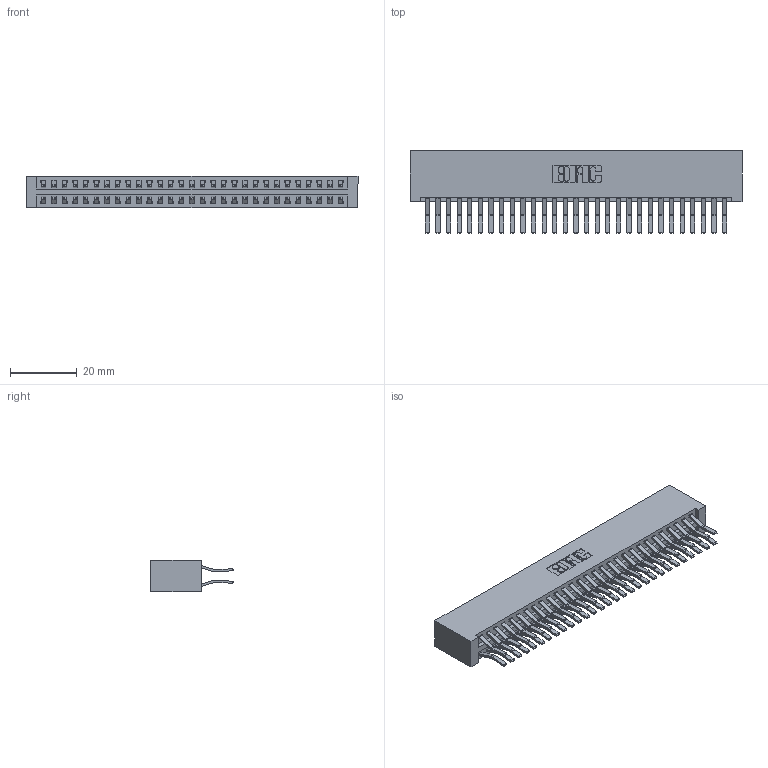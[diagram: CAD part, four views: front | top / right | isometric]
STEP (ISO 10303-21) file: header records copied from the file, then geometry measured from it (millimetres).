
FILE_DESCRIPTION (( 'STEP AP203' ), '1' );
FILE_NAME ('346-058-560-201.STEP', '2022-05-21T09:47:39', ( '' ), ( '' ), 'SwSTEP 2.0', 'SolidWorks 2020', '' );
FILE_SCHEMA (( 'CONFIG_CONTROL_DESIGN' ));
Length unit declared in the file: inch
Products named in the file (3): 346-058-560-201; 345-292-001_560 Tail; 346 Part_No Mounting Lugs
Assembly tree (59 placements, depth 2):
  346-058-560-201
    346 Part_No Mounting Lugs
    345-292-001_560 Tail  x58
Bounding box: 99.31 x 24.78 x 9.4 mm (x, y, z)
Volume: 10536.8 mm3; surface area: 15456.7 mm2
Topology: 59 solids, 59 shells, 3246 faces, 9643 edges, 6350 vertices
Faces by surface type: plane 2102, cylinder 1144
Entity records: 20487 total; most frequent: CARTESIAN_POINT 3392, ORIENTED_EDGE 3326, DIRECTION 3039, EDGE_CURVE 1663, LINE 1419, VECTOR 1419, VERTEX_POINT 1106, AXIS2_PLACEMENT_3D 810
